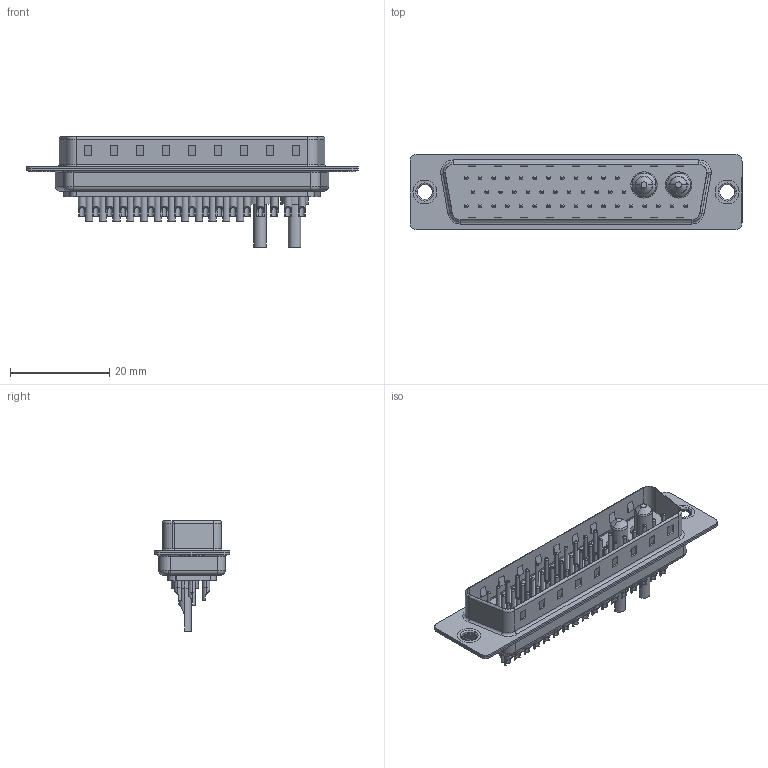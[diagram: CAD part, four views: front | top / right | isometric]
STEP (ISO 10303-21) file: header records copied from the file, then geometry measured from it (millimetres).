
FILE_DESCRIPTION (( 'STEP AP203' ), '1' );
FILE_NAME ('627-43W2222-1N1.STEP', '2019-06-19T20:59:15', ( '' ), ( '' ), 'SwSTEP 2.0', 'SolidWorks 2016', '' );
FILE_SCHEMA (( 'CONFIG_CONTROL_DESIGN' ));
Length unit declared in the file: millimetre
Products named in the file (9): 627Combo Thru Hole Rivet; Power Pin_10A SC; 627Combo Contact Row 1_22; 627Combo Contact Row 2_22L; 627Combo Contact Row 3_22; 627-43W2222-1N1; 627Combo Housing_43W2; 627Combo Shell Rear_50 Contacts; 627Combo Shell Front_50 Contacts
Assembly tree (48 placements, depth 2):
  627-43W2222-1N1
    627Combo Housing_43W2
    627Combo Shell Rear_50 Contacts
    627Combo Shell Front_50 Contacts
    627Combo Thru Hole Rivet  x2
    Power Pin_10A SC  x2
    627Combo Contact Row 1_22  x12
    627Combo Contact Row 2_22L  x12
    627Combo Contact Row 3_22  x17
Bounding box: 67 x 15.3 x 22.3 mm (x, y, z)
Volume: 4664.8 mm3; surface area: 11069 mm2
Topology: 50 solids, 50 shells, 1993 faces, 4617 edges, 2819 vertices
Faces by surface type: cylinder 825, plane 596, torus 472, cone 96, bspline 4
Entity records: 26845 total; most frequent: DIRECTION 4634, CARTESIAN_POINT 4393, ORIENTED_EDGE 3944, EDGE_CURVE 1972, AXIS2_PLACEMENT_3D 1833, VERTEX_POINT 1262, EDGE_LOOP 1070, VECTOR 968
